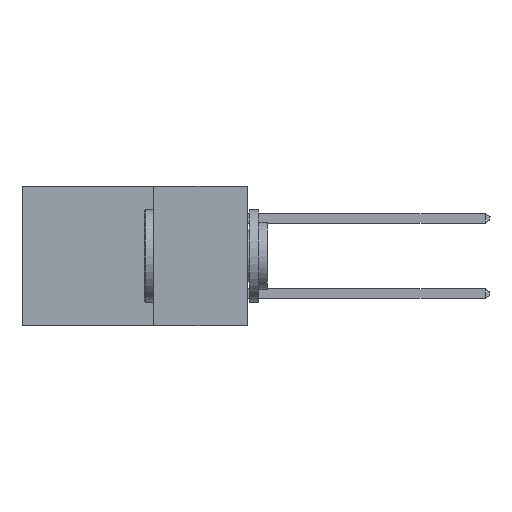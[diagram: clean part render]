
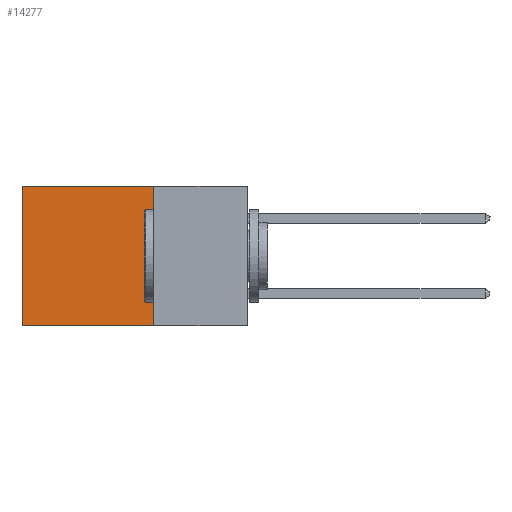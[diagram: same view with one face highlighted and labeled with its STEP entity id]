
A CAD part, left-side view. The second image highlights one B-rep face of the part: STEP entity #14277.
In plain terms, the highlighted planar face has unit normal (-1, 0, 0).
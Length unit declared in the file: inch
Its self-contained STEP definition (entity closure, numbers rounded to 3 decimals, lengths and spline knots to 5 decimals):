
#308 = CARTESIAN_POINT ( 'NONE',  ( 0.2615, 0.6, 0. ) ) ;
#692 = CARTESIAN_POINT ( 'NONE',  ( 0.2615, 0.25, -0.37 ) ) ;
#1678 = DIRECTION ( 'NONE',  ( 0., 0., -1. ) ) ;
#2209 = CARTESIAN_POINT ( 'NONE',  ( 0.2615, 0.25, 0. ) ) ;
#2407 = PLANE ( 'NONE',  #8523 ) ;
#2562 = CARTESIAN_POINT ( 'NONE',  ( 0.2615, 0.25, -0.37 ) ) ;
#2595 = LINE ( 'NONE', #12047, #8200 ) ;
#3233 = ORIENTED_EDGE ( 'NONE', *, *, #6243, .F. ) ;
#3944 = FACE_OUTER_BOUND ( 'NONE', #13647, .T. ) ;
#5375 = VERTEX_POINT ( 'NONE', #308 ) ;
#5797 = CARTESIAN_POINT ( 'NONE',  ( 0.2615, 0.25, -0.37 ) ) ;
#6198 = VECTOR ( 'NONE', #1678, 39.37008 ) ;
#6243 = EDGE_CURVE ( 'NONE', #14646, #17047, #11906, .T. ) ;
#7956 = VERTEX_POINT ( 'NONE', #15047 ) ;
#8200 = VECTOR ( 'NONE', #14791, 39.37008 ) ;
#8523 = AXIS2_PLACEMENT_3D ( 'NONE', #14677, #17670, #13568 ) ;
#9325 = ORIENTED_EDGE ( 'NONE', *, *, #17781, .F. ) ;
#9598 = ORIENTED_EDGE ( 'NONE', *, *, #12407, .T. ) ;
#9924 = LINE ( 'NONE', #15503, #6198 ) ;
#11183 = ORIENTED_EDGE ( 'NONE', *, *, #14018, .T. ) ;
#11906 = LINE ( 'NONE', #2562, #16689 ) ;
#12047 = CARTESIAN_POINT ( 'NONE',  ( 0.2615, 0.25, 0. ) ) ;
#12407 = EDGE_CURVE ( 'NONE', #14646, #5375, #2595, .T. ) ;
#12616 = LINE ( 'NONE', #5797, #15398 ) ;
#13568 = DIRECTION ( 'NONE',  ( 0., 0., -1. ) ) ;
#13647 = EDGE_LOOP ( 'NONE', ( #11183, #9325, #3233, #9598 ) ) ;
#14018 = EDGE_CURVE ( 'NONE', #5375, #7956, #9924, .T. ) ;
#14277 = ADVANCED_FACE ( 'NONE', ( #3944 ), #2407, .F. ) ;
#14646 = VERTEX_POINT ( 'NONE', #2209 ) ;
#14677 = CARTESIAN_POINT ( 'NONE',  ( 0.2615, 0.25, -0.37 ) ) ;
#14791 = DIRECTION ( 'NONE',  ( 0., 1., 0. ) ) ;
#15047 = CARTESIAN_POINT ( 'NONE',  ( 0.2615, 0.6, -0.37 ) ) ;
#15398 = VECTOR ( 'NONE', #16814, 39.37008 ) ;
#15503 = CARTESIAN_POINT ( 'NONE',  ( 0.2615, 0.6, -0.37 ) ) ;
#16689 = VECTOR ( 'NONE', #17833, 39.37008 ) ;
#16814 = DIRECTION ( 'NONE',  ( 0., 1., 0. ) ) ;
#17047 = VERTEX_POINT ( 'NONE', #692 ) ;
#17670 = DIRECTION ( 'NONE',  ( 1., 0., 0. ) ) ;
#17781 = EDGE_CURVE ( 'NONE', #17047, #7956, #12616, .T. ) ;
#17833 = DIRECTION ( 'NONE',  ( 0., 0., -1. ) ) ;
